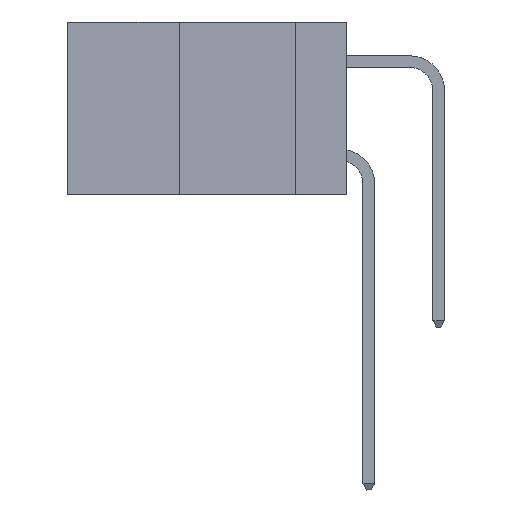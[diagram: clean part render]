
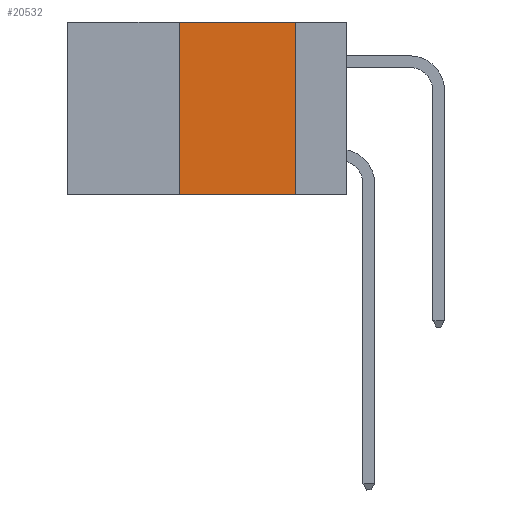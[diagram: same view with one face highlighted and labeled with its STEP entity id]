
A CAD part, left-side view. The second image highlights one B-rep face of the part: STEP entity #20532.
In plain terms, the highlighted planar face has unit normal (-1, 0, 0).
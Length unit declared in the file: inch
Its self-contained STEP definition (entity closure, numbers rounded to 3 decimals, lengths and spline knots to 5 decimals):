
#654 = LINE ( 'NONE', #15057, #5361 ) ;
#1196 = ORIENTED_EDGE ( 'NONE', *, *, #12901, .F. ) ;
#2330 = VECTOR ( 'NONE', #18469, 39.37008 ) ;
#3074 = ORIENTED_EDGE ( 'NONE', *, *, #16484, .F. ) ;
#3253 = VERTEX_POINT ( 'NONE', #21045 ) ;
#3335 = DIRECTION ( 'NONE',  ( 0., 0., -1. ) ) ;
#4076 = DIRECTION ( 'NONE',  ( 0., 0., -1. ) ) ;
#4317 = CARTESIAN_POINT ( 'NONE',  ( 0., 0.11, 0. ) ) ;
#4826 = CARTESIAN_POINT ( 'NONE',  ( 0., 0.36, 0. ) ) ;
#5361 = VECTOR ( 'NONE', #17538, 39.37008 ) ;
#5957 = LINE ( 'NONE', #4317, #17296 ) ;
#6566 = ORIENTED_EDGE ( 'NONE', *, *, #12225, .F. ) ;
#8141 = CARTESIAN_POINT ( 'NONE',  ( 0., 0.6, 0. ) ) ;
#8511 = CARTESIAN_POINT ( 'NONE',  ( 0., 0.36, 0. ) ) ;
#9926 = DIRECTION ( 'NONE',  ( 1., 0., 0. ) ) ;
#10041 = CARTESIAN_POINT ( 'NONE',  ( 0., 0.36, -0.37 ) ) ;
#12225 = EDGE_CURVE ( 'NONE', #14664, #21767, #16841, .T. ) ;
#12498 = EDGE_LOOP ( 'NONE', ( #3074, #1196, #6566, #12690 ) ) ;
#12690 = ORIENTED_EDGE ( 'NONE', *, *, #18628, .T. ) ;
#12871 = CARTESIAN_POINT ( 'NONE',  ( 0., 0.11, 0. ) ) ;
#12901 = EDGE_CURVE ( 'NONE', #21767, #18203, #13143, .T. ) ;
#13143 = LINE ( 'NONE', #18329, #2330 ) ;
#13224 = FACE_OUTER_BOUND ( 'NONE', #12498, .T. ) ;
#13582 = AXIS2_PLACEMENT_3D ( 'NONE', #8141, #9926, #3335 ) ;
#13825 = DIRECTION ( 'NONE',  ( 0., 0., 1. ) ) ;
#14664 = VERTEX_POINT ( 'NONE', #10041 ) ;
#15057 = CARTESIAN_POINT ( 'NONE',  ( 0., 0.6, -0.37 ) ) ;
#16484 = EDGE_CURVE ( 'NONE', #18203, #3253, #5957, .T. ) ;
#16841 = LINE ( 'NONE', #8511, #18411 ) ;
#17296 = VECTOR ( 'NONE', #4076, 39.37008 ) ;
#17538 = DIRECTION ( 'NONE',  ( 0., -1., 0. ) ) ;
#18203 = VERTEX_POINT ( 'NONE', #12871 ) ;
#18329 = CARTESIAN_POINT ( 'NONE',  ( 0., 0.6, 0. ) ) ;
#18411 = VECTOR ( 'NONE', #13825, 39.37008 ) ;
#18469 = DIRECTION ( 'NONE',  ( 0., -1., 0. ) ) ;
#18628 = EDGE_CURVE ( 'NONE', #14664, #3253, #654, .T. ) ;
#19821 = PLANE ( 'NONE',  #13582 ) ;
#20532 = ADVANCED_FACE ( 'NONE', ( #13224 ), #19821, .F. ) ;
#21045 = CARTESIAN_POINT ( 'NONE',  ( 0., 0.11, -0.37 ) ) ;
#21767 = VERTEX_POINT ( 'NONE', #4826 ) ;
